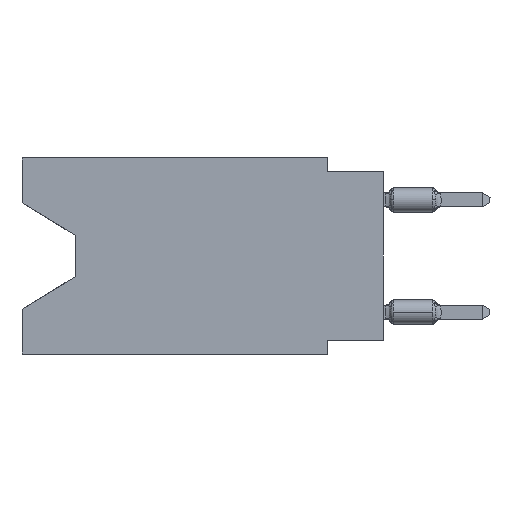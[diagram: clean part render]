
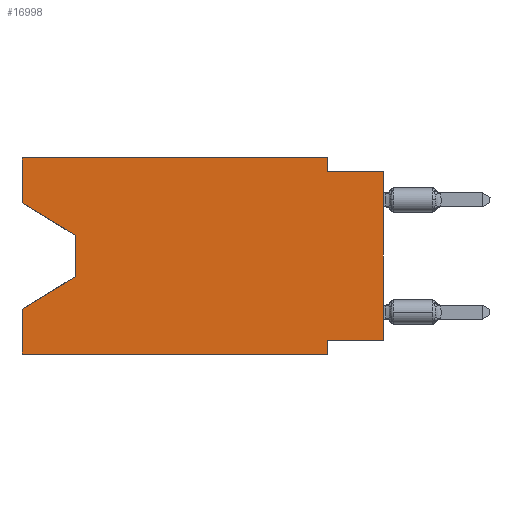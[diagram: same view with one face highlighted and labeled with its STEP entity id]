
A CAD part, left-side view. The second image highlights one B-rep face of the part: STEP entity #16998.
In plain terms, the highlighted planar face has unit normal (-1, 0, 0).
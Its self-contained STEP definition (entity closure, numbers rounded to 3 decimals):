
#123 = CARTESIAN_POINT ( 'NONE',  ( 0., 13.97, -5.385 ) ) ;
#191 = VECTOR ( 'NONE', #17618, 1000. ) ;
#556 = VECTOR ( 'NONE', #1304, 1000. ) ;
#709 = CARTESIAN_POINT ( 'NONE',  ( 0., 0., -8.255 ) ) ;
#1102 = DIRECTION ( 'NONE',  ( 0., 0., 1. ) ) ;
#1258 = CARTESIAN_POINT ( 'NONE',  ( 0., 2.54, 0. ) ) ;
#1304 = DIRECTION ( 'NONE',  ( 0., 0.855, -0.519 ) ) ;
#1412 = CARTESIAN_POINT ( 'NONE',  ( 0., 2.54, -8.89 ) ) ;
#1451 = VECTOR ( 'NONE', #19316, 1000. ) ;
#2144 = AXIS2_PLACEMENT_3D ( 'NONE', #3074, #17412, #5238 ) ;
#2185 = EDGE_CURVE ( 'NONE', #24372, #26678, #18075, .T. ) ;
#2245 = EDGE_CURVE ( 'NONE', #9731, #26678, #24717, .T. ) ;
#3074 = CARTESIAN_POINT ( 'NONE',  ( 0., 16.383, 0. ) ) ;
#3274 = EDGE_CURVE ( 'NONE', #22415, #21939, #30085, .T. ) ;
#3388 = EDGE_CURVE ( 'NONE', #14207, #16874, #12319, .T. ) ;
#3527 = CARTESIAN_POINT ( 'NONE',  ( 0., 2.54, 0. ) ) ;
#3583 = DIRECTION ( 'NONE',  ( 0., -1., 0. ) ) ;
#3955 = EDGE_CURVE ( 'NONE', #7492, #18334, #29405, .T. ) ;
#4311 = CARTESIAN_POINT ( 'NONE',  ( 0., 16.383, 0. ) ) ;
#4321 = VECTOR ( 'NONE', #22551, 1000. ) ;
#5030 = CARTESIAN_POINT ( 'NONE',  ( 0., 16.383, -2.038 ) ) ;
#5194 = DIRECTION ( 'NONE',  ( 0., 1., 0. ) ) ;
#5238 = DIRECTION ( 'NONE',  ( 0., 0., -1. ) ) ;
#5835 = PLANE ( 'NONE',  #2144 ) ;
#6051 = LINE ( 'NONE', #19645, #26029 ) ;
#6662 = DIRECTION ( 'NONE',  ( 0., -0.855, -0.519 ) ) ;
#7026 = ORIENTED_EDGE ( 'NONE', *, *, #21772, .F. ) ;
#7492 = VERTEX_POINT ( 'NONE', #123 ) ;
#7693 = ORIENTED_EDGE ( 'NONE', *, *, #3955, .T. ) ;
#8366 = CARTESIAN_POINT ( 'NONE',  ( 0., 13.97, -3.505 ) ) ;
#8480 = EDGE_CURVE ( 'NONE', #11438, #16874, #15015, .T. ) ;
#8512 = LINE ( 'NONE', #1258, #4321 ) ;
#9316 = EDGE_CURVE ( 'NONE', #11438, #24372, #28961, .T. ) ;
#9552 = DIRECTION ( 'NONE',  ( 0., 0., 1. ) ) ;
#9634 = DIRECTION ( 'NONE',  ( 0., 0., 1. ) ) ;
#9720 = ORIENTED_EDGE ( 'NONE', *, *, #11052, .F. ) ;
#9731 = VERTEX_POINT ( 'NONE', #19344 ) ;
#9892 = VERTEX_POINT ( 'NONE', #8366 ) ;
#10013 = CARTESIAN_POINT ( 'NONE',  ( 0., 0., -0.635 ) ) ;
#10511 = VECTOR ( 'NONE', #6662, 1000. ) ;
#10864 = CARTESIAN_POINT ( 'NONE',  ( 0., 13.97, -5.385 ) ) ;
#11027 = LINE ( 'NONE', #20442, #1451 ) ;
#11052 = EDGE_CURVE ( 'NONE', #18327, #14207, #8512, .T. ) ;
#11118 = EDGE_CURVE ( 'NONE', #9731, #18334, #6051, .T. ) ;
#11438 = VERTEX_POINT ( 'NONE', #14375 ) ;
#11839 = VECTOR ( 'NONE', #26819, 1000. ) ;
#12016 = VECTOR ( 'NONE', #3583, 1000. ) ;
#12150 = CARTESIAN_POINT ( 'NONE',  ( 0., 16.383, 0. ) ) ;
#12319 = LINE ( 'NONE', #10013, #11839 ) ;
#13008 = ORIENTED_EDGE ( 'NONE', *, *, #11118, .F. ) ;
#13235 = CARTESIAN_POINT ( 'NONE',  ( 0., 2.54, -0.635 ) ) ;
#14207 = VERTEX_POINT ( 'NONE', #13235 ) ;
#14375 = CARTESIAN_POINT ( 'NONE',  ( 0., 0., -8.255 ) ) ;
#15015 = LINE ( 'NONE', #24424, #20747 ) ;
#15466 = CARTESIAN_POINT ( 'NONE',  ( 0., 16.383, -8.89 ) ) ;
#15626 = CARTESIAN_POINT ( 'NONE',  ( 0., 16.383, -2.038 ) ) ;
#16245 = ORIENTED_EDGE ( 'NONE', *, *, #2185, .F. ) ;
#16342 = EDGE_CURVE ( 'NONE', #22415, #9892, #20699, .T. ) ;
#16874 = VERTEX_POINT ( 'NONE', #28547 ) ;
#16998 = ADVANCED_FACE ( 'NONE', ( #29150 ), #5835, .F. ) ;
#17412 = DIRECTION ( 'NONE',  ( 1., 0., 0. ) ) ;
#17618 = DIRECTION ( 'NONE',  ( 0., 0., -1. ) ) ;
#18075 = LINE ( 'NONE', #1412, #191 ) ;
#18327 = VERTEX_POINT ( 'NONE', #3527 ) ;
#18334 = VERTEX_POINT ( 'NONE', #29014 ) ;
#19316 = DIRECTION ( 'NONE',  ( 0., 0., -1. ) ) ;
#19344 = CARTESIAN_POINT ( 'NONE',  ( 0., 16.383, -8.89 ) ) ;
#19505 = ORIENTED_EDGE ( 'NONE', *, *, #16342, .T. ) ;
#19645 = CARTESIAN_POINT ( 'NONE',  ( 0., 16.383, 0. ) ) ;
#19748 = ORIENTED_EDGE ( 'NONE', *, *, #3274, .F. ) ;
#19807 = VECTOR ( 'NONE', #5194, 1000. ) ;
#19871 = EDGE_CURVE ( 'NONE', #9892, #7492, #11027, .T. ) ;
#19997 = VECTOR ( 'NONE', #29059, 1000. ) ;
#20442 = CARTESIAN_POINT ( 'NONE',  ( 0., 13.97, -3.505 ) ) ;
#20699 = LINE ( 'NONE', #15626, #10511 ) ;
#20747 = VECTOR ( 'NONE', #9634, 1000. ) ;
#21772 = EDGE_CURVE ( 'NONE', #21939, #18327, #26871, .T. ) ;
#21939 = VERTEX_POINT ( 'NONE', #12150 ) ;
#22415 = VERTEX_POINT ( 'NONE', #5030 ) ;
#22551 = DIRECTION ( 'NONE',  ( 0., 0., -1. ) ) ;
#22810 = ORIENTED_EDGE ( 'NONE', *, *, #3388, .F. ) ;
#23031 = ORIENTED_EDGE ( 'NONE', *, *, #9316, .F. ) ;
#23720 = CARTESIAN_POINT ( 'NONE',  ( 0., 2.54, -8.89 ) ) ;
#24027 = ORIENTED_EDGE ( 'NONE', *, *, #2245, .T. ) ;
#24372 = VERTEX_POINT ( 'NONE', #28254 ) ;
#24424 = CARTESIAN_POINT ( 'NONE',  ( 0., 0., 0. ) ) ;
#24717 = LINE ( 'NONE', #15466, #12016 ) ;
#25185 = ORIENTED_EDGE ( 'NONE', *, *, #19871, .T. ) ;
#26029 = VECTOR ( 'NONE', #1102, 1000. ) ;
#26572 = CARTESIAN_POINT ( 'NONE',  ( 0., 16.383, 0. ) ) ;
#26608 = ORIENTED_EDGE ( 'NONE', *, *, #8480, .T. ) ;
#26678 = VERTEX_POINT ( 'NONE', #23720 ) ;
#26819 = DIRECTION ( 'NONE',  ( 0., -1., 0. ) ) ;
#26871 = LINE ( 'NONE', #26572, #19997 ) ;
#28254 = CARTESIAN_POINT ( 'NONE',  ( 0., 2.54, -8.255 ) ) ;
#28547 = CARTESIAN_POINT ( 'NONE',  ( 0., 0., -0.635 ) ) ;
#28610 = VECTOR ( 'NONE', #9552, 1000. ) ;
#28961 = LINE ( 'NONE', #709, #19807 ) ;
#29014 = CARTESIAN_POINT ( 'NONE',  ( 0., 16.383, -6.852 ) ) ;
#29059 = DIRECTION ( 'NONE',  ( 0., -1., 0. ) ) ;
#29150 = FACE_OUTER_BOUND ( 'NONE', #29310, .T. ) ;
#29310 = EDGE_LOOP ( 'NONE', ( #19505, #25185, #7693, #13008, #24027, #16245, #23031, #26608, #22810, #9720, #7026, #19748 ) ) ;
#29405 = LINE ( 'NONE', #10864, #556 ) ;
#30085 = LINE ( 'NONE', #4311, #28610 ) ;
